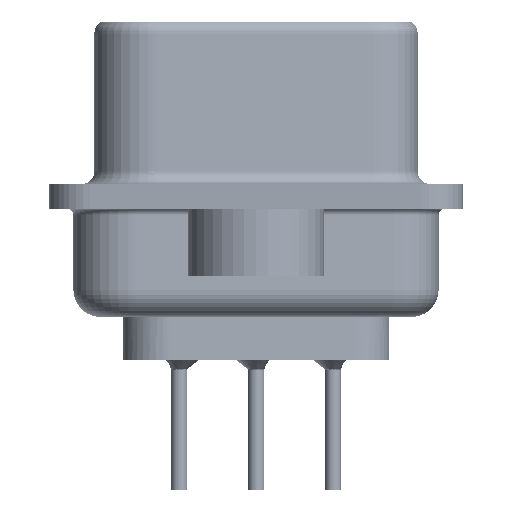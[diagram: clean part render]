
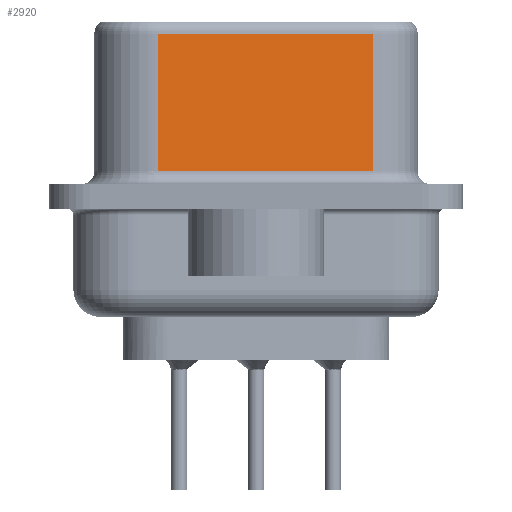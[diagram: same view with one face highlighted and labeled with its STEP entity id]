
A CAD part, left-side view. The second image highlights one B-rep face of the part: STEP entity #2920.
In plain terms, the highlighted planar face has unit normal (-0.985, -0.174, 0).
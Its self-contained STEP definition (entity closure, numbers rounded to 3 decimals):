
#436 = CARTESIAN_POINT ( 'NONE',  ( 3.73, 3.628, 0.95 ) ) ;
#1035 = EDGE_CURVE ( 'NONE', #17174, #28238, #12427, .T. ) ;
#2920 = ADVANCED_FACE ( 'NONE', ( #24839 ), #19162, .F. ) ;
#5160 = EDGE_CURVE ( 'NONE', #33640, #28660, #30051, .T. ) ;
#7030 = CARTESIAN_POINT ( 'NONE',  ( 5.132, -4.322, 6.52 ) ) ;
#7558 = LINE ( 'NONE', #7030, #35787 ) ;
#7722 = CARTESIAN_POINT ( 'NONE',  ( 5.132, -4.322, 6.52 ) ) ;
#8039 = ORIENTED_EDGE ( 'NONE', *, *, #1035, .T. ) ;
#8172 = CARTESIAN_POINT ( 'NONE',  ( 5.132, -4.322, 6.02 ) ) ;
#8886 = CARTESIAN_POINT ( 'NONE',  ( 3.73, 3.628, 6.52 ) ) ;
#9919 = CARTESIAN_POINT ( 'NONE',  ( 5.132, -4.322, 6.02 ) ) ;
#10324 = EDGE_CURVE ( 'NONE', #33640, #28238, #7558, .T. ) ;
#11910 = DIRECTION ( 'NONE',  ( 0.174, -0.985, 0. ) ) ;
#12199 = CARTESIAN_POINT ( 'NONE',  ( 3.73, 3.628, 6.02 ) ) ;
#12427 = LINE ( 'NONE', #25941, #33167 ) ;
#13947 = LINE ( 'NONE', #8886, #14117 ) ;
#14117 = VECTOR ( 'NONE', #19970, 1000. ) ;
#16165 = DIRECTION ( 'NONE',  ( -0.174, 0.985, 0. ) ) ;
#17174 = VERTEX_POINT ( 'NONE', #436 ) ;
#18828 = DIRECTION ( 'NONE',  ( 0.985, 0.174, 0. ) ) ;
#19162 = PLANE ( 'NONE',  #29944 ) ;
#19243 = ORIENTED_EDGE ( 'NONE', *, *, #5160, .T. ) ;
#19970 = DIRECTION ( 'NONE',  ( 0., 0., -1. ) ) ;
#22767 = VECTOR ( 'NONE', #16165, 1000. ) ;
#24087 = ORIENTED_EDGE ( 'NONE', *, *, #31640, .T. ) ;
#24367 = EDGE_LOOP ( 'NONE', ( #34844, #19243, #24087, #8039 ) ) ;
#24839 = FACE_OUTER_BOUND ( 'NONE', #24367, .T. ) ;
#25753 = CARTESIAN_POINT ( 'NONE',  ( 5.132, -4.322, 0.95 ) ) ;
#25941 = CARTESIAN_POINT ( 'NONE',  ( 5.132, -4.322, 0.95 ) ) ;
#26509 = DIRECTION ( 'NONE',  ( 0., 0., -1. ) ) ;
#27384 = DIRECTION ( 'NONE',  ( -0.174, 0.985, 0. ) ) ;
#28238 = VERTEX_POINT ( 'NONE', #25753 ) ;
#28660 = VERTEX_POINT ( 'NONE', #12199 ) ;
#29944 = AXIS2_PLACEMENT_3D ( 'NONE', #7722, #18828, #27384 ) ;
#30051 = LINE ( 'NONE', #8172, #22767 ) ;
#31640 = EDGE_CURVE ( 'NONE', #28660, #17174, #13947, .T. ) ;
#33167 = VECTOR ( 'NONE', #11910, 1000. ) ;
#33640 = VERTEX_POINT ( 'NONE', #9919 ) ;
#34844 = ORIENTED_EDGE ( 'NONE', *, *, #10324, .F. ) ;
#35787 = VECTOR ( 'NONE', #26509, 1000. ) ;
